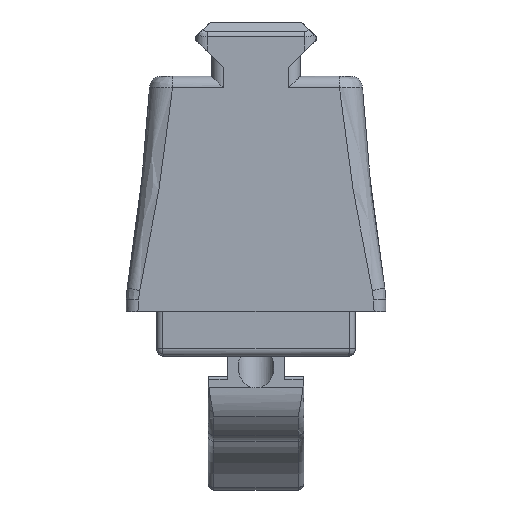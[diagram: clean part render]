
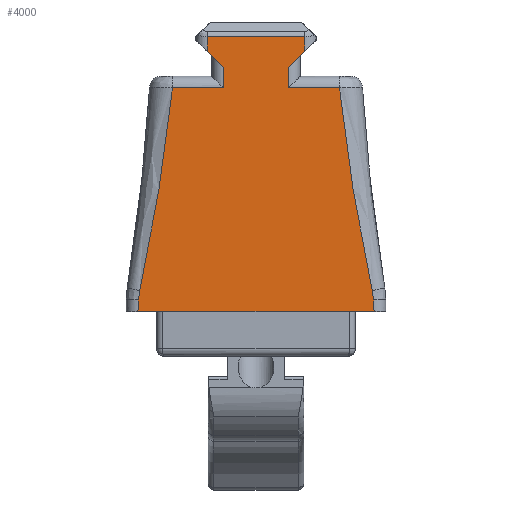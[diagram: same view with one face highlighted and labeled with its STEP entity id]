
A CAD part, top view. The second image highlights one B-rep face of the part: STEP entity #4000.
In plain terms, the highlighted planar face has unit normal (0, 0, 1).
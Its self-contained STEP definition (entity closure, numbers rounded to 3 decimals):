
#36=(
BOUNDED_CURVE()
B_SPLINE_CURVE(3,(#6213,#6214,#6215,#6216,#6217,#6218,#6219,#6220,#6221,
#6222,#6223),.UNSPECIFIED.,.F.,.F.)
B_SPLINE_CURVE_WITH_KNOTS((4,2,3,2,4),(0.358,1.277,
2.196,3.125,3.853),.UNSPECIFIED.)
CURVE()
GEOMETRIC_REPRESENTATION_ITEM()
RATIONAL_B_SPLINE_CURVE((1.,1.,1.,1.,1.,1.,1.,1.,1.,1.,1.))
REPRESENTATION_ITEM('')
);
#37=(
BOUNDED_CURVE()
B_SPLINE_CURVE(3,(#6234,#6235,#6236,#6237,#6238,#6239,#6240,#6241,#6242,
#6243,#6244),.UNSPECIFIED.,.F.,.F.)
B_SPLINE_CURVE_WITH_KNOTS((4,2,3,2,4),(0.358,1.277,
2.196,3.125,3.853),.UNSPECIFIED.)
CURVE()
GEOMETRIC_REPRESENTATION_ITEM()
RATIONAL_B_SPLINE_CURVE((1.,1.,1.,1.,1.,1.,1.,1.,1.,1.,1.))
REPRESENTATION_ITEM('')
);
#91=B_SPLINE_CURVE_WITH_KNOTS('',3,(#6246,#6247,#6248,#6249),
 .UNSPECIFIED.,.F.,.F.,(4,4),(0.195,0.358),
 .UNSPECIFIED.);
#92=B_SPLINE_CURVE_WITH_KNOTS('',3,(#6251,#6252,#6253,#6254),
 .UNSPECIFIED.,.F.,.F.,(4,4),(0.,0.195),.UNSPECIFIED.);
#93=B_SPLINE_CURVE_WITH_KNOTS('',3,(#6258,#6259,#6260,#6261),
 .UNSPECIFIED.,.F.,.F.,(4,4),(0.,0.195),.UNSPECIFIED.);
#94=B_SPLINE_CURVE_WITH_KNOTS('',3,(#6262,#6263,#6264,#6265),
 .UNSPECIFIED.,.F.,.F.,(4,4),(0.195,0.358),
 .UNSPECIFIED.);
#352=PLANE('',#4290);
#470=FACE_OUTER_BOUND('',#724,.T.);
#724=EDGE_LOOP('',(#2752,#2753,#2754,#2755,#2756,#2757,#2758,#2759,#2760,
#2761,#2762,#2763,#2764,#2765,#2766,#2767));
#963=LINE('',#5907,#1274);
#968=LINE('',#5924,#1279);
#985=LINE('',#6045,#1296);
#990=LINE('',#6232,#1301);
#991=LINE('',#6256,#1302);
#992=LINE('',#6267,#1303);
#993=LINE('',#6269,#1304);
#994=LINE('',#6271,#1305);
#995=LINE('',#6273,#1306);
#996=LINE('',#6274,#1307);
#1274=VECTOR('',#4702,10.);
#1279=VECTOR('',#4717,10.);
#1296=VECTOR('',#4792,10.);
#1301=VECTOR('',#4811,10.);
#1302=VECTOR('',#4812,10.);
#1303=VECTOR('',#4813,10.);
#1304=VECTOR('',#4814,10.);
#1305=VECTOR('',#4815,10.);
#1306=VECTOR('',#4816,10.);
#1307=VECTOR('',#4817,10.);
#1642=VERTEX_POINT('',#5900);
#1645=VERTEX_POINT('',#5905);
#1649=VERTEX_POINT('',#5917);
#1652=VERTEX_POINT('',#5922);
#1678=VERTEX_POINT('',#6041);
#1689=VERTEX_POINT('',#6212);
#1690=VERTEX_POINT('',#6231);
#1691=VERTEX_POINT('',#6233);
#1692=VERTEX_POINT('',#6245);
#1693=VERTEX_POINT('',#6250);
#1694=VERTEX_POINT('',#6255);
#1695=VERTEX_POINT('',#6257);
#1696=VERTEX_POINT('',#6266);
#1697=VERTEX_POINT('',#6268);
#1698=VERTEX_POINT('',#6270);
#1699=VERTEX_POINT('',#6272);
#2024=EDGE_CURVE('',#1645,#1642,#963,.T.);
#2032=EDGE_CURVE('',#1652,#1649,#968,.T.);
#2073=EDGE_CURVE('',#1649,#1678,#985,.T.);
#2090=EDGE_CURVE('',#1689,#1678,#36,.T.);
#2092=EDGE_CURVE('',#1690,#1645,#990,.T.);
#2093=EDGE_CURVE('',#1691,#1690,#37,.T.);
#2094=EDGE_CURVE('',#1692,#1691,#91,.T.);
#2095=EDGE_CURVE('',#1693,#1692,#92,.T.);
#2096=EDGE_CURVE('',#1693,#1694,#991,.T.);
#2097=EDGE_CURVE('',#1694,#1695,#93,.T.);
#2098=EDGE_CURVE('',#1695,#1689,#94,.T.);
#2099=EDGE_CURVE('',#1652,#1696,#992,.T.);
#2100=EDGE_CURVE('',#1697,#1696,#993,.T.);
#2101=EDGE_CURVE('',#1698,#1697,#994,.T.);
#2102=EDGE_CURVE('',#1699,#1698,#995,.T.);
#2103=EDGE_CURVE('',#1699,#1642,#996,.T.);
#2752=ORIENTED_EDGE('',*,*,#2092,.F.);
#2753=ORIENTED_EDGE('',*,*,#2093,.F.);
#2754=ORIENTED_EDGE('',*,*,#2094,.F.);
#2755=ORIENTED_EDGE('',*,*,#2095,.F.);
#2756=ORIENTED_EDGE('',*,*,#2096,.T.);
#2757=ORIENTED_EDGE('',*,*,#2097,.T.);
#2758=ORIENTED_EDGE('',*,*,#2098,.T.);
#2759=ORIENTED_EDGE('',*,*,#2090,.T.);
#2760=ORIENTED_EDGE('',*,*,#2073,.F.);
#2761=ORIENTED_EDGE('',*,*,#2032,.F.);
#2762=ORIENTED_EDGE('',*,*,#2099,.T.);
#2763=ORIENTED_EDGE('',*,*,#2100,.F.);
#2764=ORIENTED_EDGE('',*,*,#2101,.F.);
#2765=ORIENTED_EDGE('',*,*,#2102,.F.);
#2766=ORIENTED_EDGE('',*,*,#2103,.T.);
#2767=ORIENTED_EDGE('',*,*,#2024,.F.);
#4000=ADVANCED_FACE('',(#470),#352,.T.);
#4290=AXIS2_PLACEMENT_3D('',#6230,#4809,#4810);
#4702=DIRECTION('',(0.,1.,0.));
#4717=DIRECTION('',(0.,-1.,0.));
#4792=DIRECTION('',(1.,0.,0.));
#4809=DIRECTION('center_axis',(0.,0.,1.));
#4810=DIRECTION('ref_axis',(1.,0.,0.));
#4811=DIRECTION('',(1.,0.,0.));
#4812=DIRECTION('',(1.,0.,0.));
#4813=DIRECTION('',(0.707,0.707,0.));
#4814=DIRECTION('',(0.,-1.,0.));
#4815=DIRECTION('',(1.,0.,0.));
#4816=DIRECTION('',(0.,1.,0.));
#4817=DIRECTION('',(0.707,-0.707,0.));
#5900=CARTESIAN_POINT('',(10.461,192.492,-108.589));
#5905=CARTESIAN_POINT('',(10.461,189.,-108.589));
#5907=CARTESIAN_POINT('',(10.461,172.867,-108.589));
#5917=CARTESIAN_POINT('',(21.492,189.,-108.589));
#5922=CARTESIAN_POINT('',(21.492,192.492,-108.589));
#5924=CARTESIAN_POINT('',(21.492,172.867,-108.589));
#6041=CARTESIAN_POINT('',(30.168,189.,-108.589));
#6045=CARTESIAN_POINT('',(5.828,189.,-108.589));
#6212=CARTESIAN_POINT('',(35.742,154.562,-108.589));
#6213=CARTESIAN_POINT('Ctrl Pts',(35.742,154.562,-108.589));
#6214=CARTESIAN_POINT('Ctrl Pts',(35.09,157.551,-108.589));
#6215=CARTESIAN_POINT('Ctrl Pts',(34.482,160.549,-108.589));
#6216=CARTESIAN_POINT('Ctrl Pts',(33.349,166.561,-108.589));
#6217=CARTESIAN_POINT('Ctrl Pts',(32.826,169.576,-108.589));
#6218=CARTESIAN_POINT('Ctrl Pts',(32.346,172.597,-108.589));
#6219=CARTESIAN_POINT('Ctrl Pts',(31.86,175.652,-108.589));
#6220=CARTESIAN_POINT('Ctrl Pts',(31.419,178.714,-108.589));
#6221=CARTESIAN_POINT('Ctrl Pts',(30.71,184.184,-108.589));
#6222=CARTESIAN_POINT('Ctrl Pts',(30.426,186.59,-108.589));
#6223=CARTESIAN_POINT('Ctrl Pts',(30.168,189.,-108.589));
#6230=CARTESIAN_POINT('Origin',(-4.32,151.,-108.589));
#6231=CARTESIAN_POINT('',(1.785,189.,-108.589));
#6232=CARTESIAN_POINT('',(5.828,189.,-108.589));
#6233=CARTESIAN_POINT('',(-3.789,154.562,-108.589));
#6234=CARTESIAN_POINT('Ctrl Pts',(-3.789,154.562,-108.589));
#6235=CARTESIAN_POINT('Ctrl Pts',(-3.137,157.551,-108.589));
#6236=CARTESIAN_POINT('Ctrl Pts',(-2.528,160.549,-108.589));
#6237=CARTESIAN_POINT('Ctrl Pts',(-1.396,166.561,-108.589));
#6238=CARTESIAN_POINT('Ctrl Pts',(-0.873,169.576,-108.589));
#6239=CARTESIAN_POINT('Ctrl Pts',(-0.393,172.597,-108.589));
#6240=CARTESIAN_POINT('Ctrl Pts',(0.093,175.652,-108.589));
#6241=CARTESIAN_POINT('Ctrl Pts',(0.534,178.714,-108.589));
#6242=CARTESIAN_POINT('Ctrl Pts',(1.243,184.184,-108.589));
#6243=CARTESIAN_POINT('Ctrl Pts',(1.528,186.59,-108.589));
#6244=CARTESIAN_POINT('Ctrl Pts',(1.785,189.,-108.589));
#6245=CARTESIAN_POINT('',(-4.003,152.949,-108.589));
#6246=CARTESIAN_POINT('Ctrl Pts',(-4.003,152.949,-108.589));
#6247=CARTESIAN_POINT('Ctrl Pts',(-3.976,153.491,-108.589));
#6248=CARTESIAN_POINT('Ctrl Pts',(-3.905,154.031,-108.589));
#6249=CARTESIAN_POINT('Ctrl Pts',(-3.789,154.562,-108.589));
#6250=CARTESIAN_POINT('',(-4.1,151.,-108.589));
#6251=CARTESIAN_POINT('Ctrl Pts',(-4.1,151.,-108.589));
#6252=CARTESIAN_POINT('Ctrl Pts',(-4.068,151.65,-108.589));
#6253=CARTESIAN_POINT('Ctrl Pts',(-4.035,152.299,-108.589));
#6254=CARTESIAN_POINT('Ctrl Pts',(-4.003,152.949,-108.589));
#6255=CARTESIAN_POINT('',(36.053,151.,-108.589));
#6256=CARTESIAN_POINT('',(15.077,151.,-108.589));
#6257=CARTESIAN_POINT('',(35.956,152.949,-108.589));
#6258=CARTESIAN_POINT('Ctrl Pts',(36.053,151.,-108.589));
#6259=CARTESIAN_POINT('Ctrl Pts',(36.021,151.65,-108.589));
#6260=CARTESIAN_POINT('Ctrl Pts',(35.989,152.299,-108.589));
#6261=CARTESIAN_POINT('Ctrl Pts',(35.956,152.949,-108.589));
#6262=CARTESIAN_POINT('Ctrl Pts',(35.956,152.949,-108.589));
#6263=CARTESIAN_POINT('Ctrl Pts',(35.929,153.491,-108.589));
#6264=CARTESIAN_POINT('Ctrl Pts',(35.858,154.031,-108.589));
#6265=CARTESIAN_POINT('Ctrl Pts',(35.742,154.562,-108.589));
#6266=CARTESIAN_POINT('',(24.261,195.261,-108.589));
#6267=CARTESIAN_POINT('',(7.051,178.051,-108.589));
#6268=CARTESIAN_POINT('',(24.261,197.704,-108.589));
#6269=CARTESIAN_POINT('',(24.261,174.397,-108.589));
#6270=CARTESIAN_POINT('',(7.692,197.704,-108.589));
#6271=CARTESIAN_POINT('',(-1.345,197.704,-108.589));
#6272=CARTESIAN_POINT('',(7.692,195.261,-108.589));
#6273=CARTESIAN_POINT('',(7.692,174.397,-108.589));
#6274=CARTESIAN_POINT('',(14.754,188.199,-108.589));
